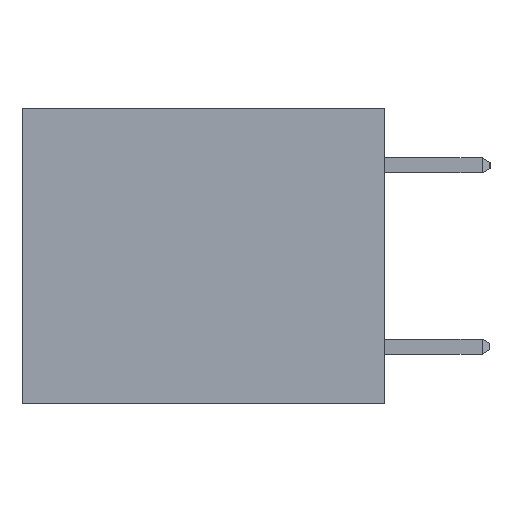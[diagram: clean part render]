
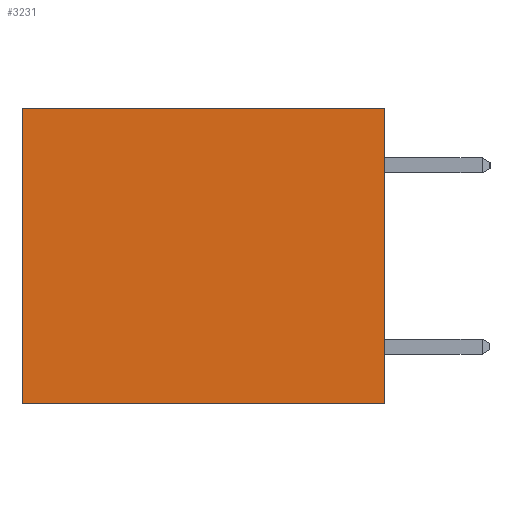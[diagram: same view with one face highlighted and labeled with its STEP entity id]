
A CAD part, left-side view. The second image highlights one B-rep face of the part: STEP entity #3231.
In plain terms, the highlighted planar face has unit normal (-1, 0, 0).
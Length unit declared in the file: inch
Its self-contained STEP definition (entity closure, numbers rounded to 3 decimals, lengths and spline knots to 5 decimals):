
#298 = DIRECTION ( 'NONE',  ( 0., 1., 0. ) ) ;
#346 = EDGE_CURVE ( 'NONE', #12612, #19634, #7488, .T. ) ;
#2156 = EDGE_LOOP ( 'NONE', ( #12052, #6439, #9284, #4891 ) ) ;
#2518 = FACE_OUTER_BOUND ( 'NONE', #2156, .T. ) ;
#2711 = CARTESIAN_POINT ( 'NONE',  ( 0.3165, 0., -0.49 ) ) ;
#3231 = ADVANCED_FACE ( 'NONE', ( #2518 ), #14700, .F. ) ;
#3345 = CARTESIAN_POINT ( 'NONE',  ( 0.3165, 0., -0.49 ) ) ;
#3997 = CARTESIAN_POINT ( 'NONE',  ( 0.3165, 0., 0. ) ) ;
#4263 = DIRECTION ( 'NONE',  ( 0., 0., -1. ) ) ;
#4594 = LINE ( 'NONE', #3345, #9933 ) ;
#4891 = ORIENTED_EDGE ( 'NONE', *, *, #14894, .T. ) ;
#5089 = EDGE_CURVE ( 'NONE', #19634, #18462, #4594, .T. ) ;
#5785 = VECTOR ( 'NONE', #8787, 39.37008 ) ;
#6036 = EDGE_CURVE ( 'NONE', #15993, #18462, #7247, .T. ) ;
#6402 = AXIS2_PLACEMENT_3D ( 'NONE', #2711, #13556, #4263 ) ;
#6439 = ORIENTED_EDGE ( 'NONE', *, *, #5089, .F. ) ;
#7247 = LINE ( 'NONE', #13405, #5785 ) ;
#7488 = LINE ( 'NONE', #15795, #16946 ) ;
#7968 = LINE ( 'NONE', #3997, #16986 ) ;
#8188 = CARTESIAN_POINT ( 'NONE',  ( 0.3165, 0.6, -0.49 ) ) ;
#8787 = DIRECTION ( 'NONE',  ( 0., 0., -1. ) ) ;
#9284 = ORIENTED_EDGE ( 'NONE', *, *, #346, .F. ) ;
#9933 = VECTOR ( 'NONE', #298, 39.37008 ) ;
#12052 = ORIENTED_EDGE ( 'NONE', *, *, #6036, .T. ) ;
#12612 = VERTEX_POINT ( 'NONE', #15242 ) ;
#12614 = CARTESIAN_POINT ( 'NONE',  ( 0.3165, 0.6, 0. ) ) ;
#13174 = DIRECTION ( 'NONE',  ( 0., 1., 0. ) ) ;
#13405 = CARTESIAN_POINT ( 'NONE',  ( 0.3165, 0.6, -0.49 ) ) ;
#13556 = DIRECTION ( 'NONE',  ( 1., 0., 0. ) ) ;
#14042 = DIRECTION ( 'NONE',  ( 0., 0., -1. ) ) ;
#14700 = PLANE ( 'NONE',  #6402 ) ;
#14894 = EDGE_CURVE ( 'NONE', #12612, #15993, #7968, .T. ) ;
#15046 = CARTESIAN_POINT ( 'NONE',  ( 0.3165, 0., -0.49 ) ) ;
#15242 = CARTESIAN_POINT ( 'NONE',  ( 0.3165, 0., 0. ) ) ;
#15795 = CARTESIAN_POINT ( 'NONE',  ( 0.3165, 0., -0.49 ) ) ;
#15993 = VERTEX_POINT ( 'NONE', #12614 ) ;
#16946 = VECTOR ( 'NONE', #14042, 39.37008 ) ;
#16986 = VECTOR ( 'NONE', #13174, 39.37008 ) ;
#18462 = VERTEX_POINT ( 'NONE', #8188 ) ;
#19634 = VERTEX_POINT ( 'NONE', #15046 ) ;
